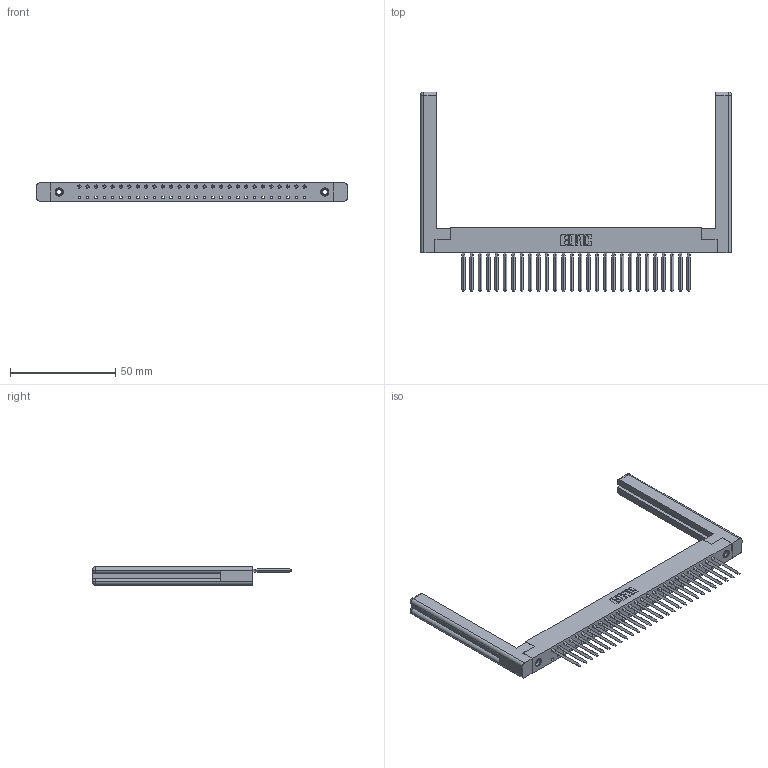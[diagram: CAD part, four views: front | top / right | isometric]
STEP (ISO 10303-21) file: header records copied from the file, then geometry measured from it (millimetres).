
FILE_DESCRIPTION (( 'STEP AP203' ), '1' );
FILE_NAME ('338-028-541-178.STEP', '2020-03-24T18:03:41', ( '' ), ( '' ), 'SwSTEP 2.0', 'SolidWorks 2016', '' );
FILE_SCHEMA (( 'CONFIG_CONTROL_DESIGN' ));
Length unit declared in the file: inch
Products named in the file (5): 338-210-001_338-210-028-004; 338-028-541-178; 345-250-001_345-250-001-102; 307-220-058; 338-290-001_541
Assembly tree (33 placements, depth 2):
  338-028-541-178
    338-210-001_338-210-028-004
    338-290-001_541  x28
    345-250-001_345-250-001-102  x2
    307-220-058  x2
Bounding box: 147.57 x 94.87 x 8.71 mm (x, y, z)
Volume: 17977.6 mm3; surface area: 22062.8 mm2
Topology: 33 solids, 33 shells, 2840 faces, 7801 edges, 4982 vertices
Faces by surface type: plane 1954, cylinder 750, bspline 112, cone 12, torus 12
Entity records: 57745 total; most frequent: CARTESIAN_POINT 11527, ORIENTED_EDGE 9722, DIRECTION 9100, EDGE_CURVE 4861, VECTOR 3634, LINE 3634, VERTEX_POINT 3154, AXIS2_PLACEMENT_3D 2733
